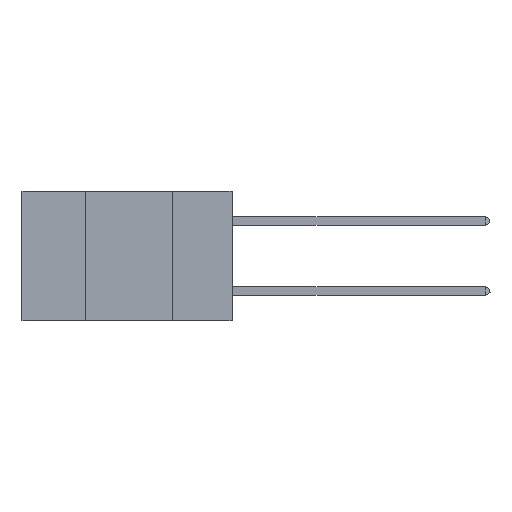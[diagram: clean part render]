
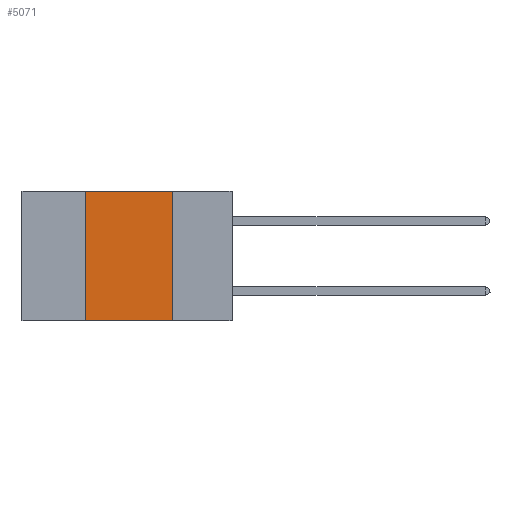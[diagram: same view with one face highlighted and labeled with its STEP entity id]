
A CAD part, left-side view. The second image highlights one B-rep face of the part: STEP entity #5071.
In plain terms, the highlighted planar face has unit normal (-1, 0, 0).
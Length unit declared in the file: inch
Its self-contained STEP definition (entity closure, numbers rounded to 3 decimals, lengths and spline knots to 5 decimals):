
#279 = CARTESIAN_POINT ( 'NONE',  ( 0., 0.42, 0. ) ) ;
#615 = VERTEX_POINT ( 'NONE', #7640 ) ;
#1637 = ORIENTED_EDGE ( 'NONE', *, *, #13843, .F. ) ;
#1852 = VERTEX_POINT ( 'NONE', #2164 ) ;
#2103 = EDGE_LOOP ( 'NONE', ( #14597, #14032, #1637, #18372 ) ) ;
#2164 = CARTESIAN_POINT ( 'NONE',  ( 0., 0.42, -0.37 ) ) ;
#2233 = AXIS2_PLACEMENT_3D ( 'NONE', #8205, #14608, #6673 ) ;
#3874 = VECTOR ( 'NONE', #4344, 39.37008 ) ;
#4344 = DIRECTION ( 'NONE',  ( 0., 0., -1. ) ) ;
#4413 = CARTESIAN_POINT ( 'NONE',  ( 0., 0.17, 0. ) ) ;
#4742 = VERTEX_POINT ( 'NONE', #10988 ) ;
#4977 = LINE ( 'NONE', #17932, #8654 ) ;
#5071 = ADVANCED_FACE ( 'NONE', ( #9492 ), #9727, .F. ) ;
#6208 = EDGE_CURVE ( 'NONE', #4742, #19043, #4977, .T. ) ;
#6673 = DIRECTION ( 'NONE',  ( 0., 0., -1. ) ) ;
#7640 = CARTESIAN_POINT ( 'NONE',  ( 0., 0.17, -0.37 ) ) ;
#8205 = CARTESIAN_POINT ( 'NONE',  ( 0., 0.6, 0. ) ) ;
#8654 = VECTOR ( 'NONE', #10156, 39.37008 ) ;
#9035 = LINE ( 'NONE', #279, #16056 ) ;
#9492 = FACE_OUTER_BOUND ( 'NONE', #2103, .T. ) ;
#9727 = PLANE ( 'NONE',  #2233 ) ;
#10156 = DIRECTION ( 'NONE',  ( 0., -1., 0. ) ) ;
#10988 = CARTESIAN_POINT ( 'NONE',  ( 0., 0.42, 0. ) ) ;
#12834 = LINE ( 'NONE', #4413, #3874 ) ;
#13843 = EDGE_CURVE ( 'NONE', #1852, #4742, #9035, .T. ) ;
#14032 = ORIENTED_EDGE ( 'NONE', *, *, #6208, .F. ) ;
#14124 = CARTESIAN_POINT ( 'NONE',  ( 0., 0.6, -0.37 ) ) ;
#14597 = ORIENTED_EDGE ( 'NONE', *, *, #16919, .F. ) ;
#14608 = DIRECTION ( 'NONE',  ( 1., 0., 0. ) ) ;
#14733 = DIRECTION ( 'NONE',  ( 0., 0., 1. ) ) ;
#14743 = VECTOR ( 'NONE', #15692, 39.37008 ) ;
#15692 = DIRECTION ( 'NONE',  ( 0., -1., 0. ) ) ;
#16056 = VECTOR ( 'NONE', #14733, 39.37008 ) ;
#16532 = LINE ( 'NONE', #14124, #14743 ) ;
#16919 = EDGE_CURVE ( 'NONE', #19043, #615, #12834, .T. ) ;
#17206 = CARTESIAN_POINT ( 'NONE',  ( 0., 0.17, 0. ) ) ;
#17932 = CARTESIAN_POINT ( 'NONE',  ( 0., 0.6, 0. ) ) ;
#18372 = ORIENTED_EDGE ( 'NONE', *, *, #19030, .T. ) ;
#19030 = EDGE_CURVE ( 'NONE', #1852, #615, #16532, .T. ) ;
#19043 = VERTEX_POINT ( 'NONE', #17206 ) ;
